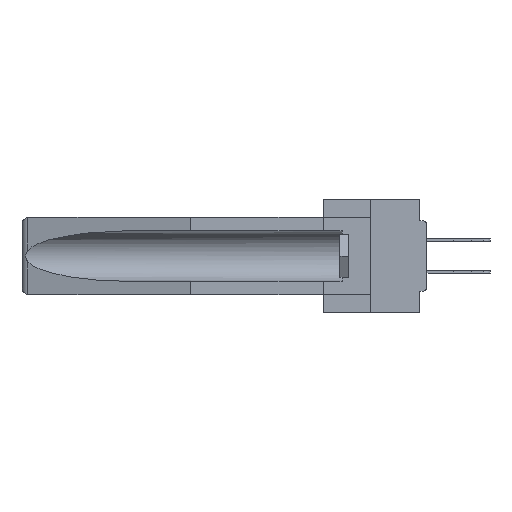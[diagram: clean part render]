
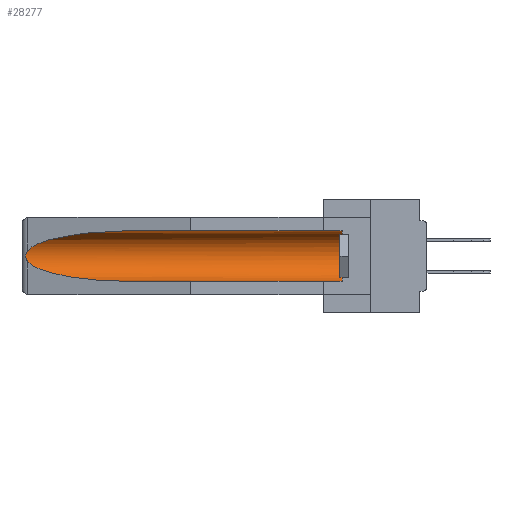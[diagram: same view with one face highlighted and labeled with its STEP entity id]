
A CAD part, left-side view. The second image highlights one B-rep face of the part: STEP entity #28277.
In plain terms, the highlighted cylindrical face has radius 2.857 mm (diameter 5.715 mm), a partial arc.
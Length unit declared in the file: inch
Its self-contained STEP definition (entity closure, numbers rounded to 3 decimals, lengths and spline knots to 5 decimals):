
#495 = ORIENTED_EDGE ( 'NONE', *, *, #36455, .T. ) ;
#780 = VERTEX_POINT ( 'NONE', #21716 ) ;
#1612 = CARTESIAN_POINT ( 'NONE',  ( 0.155, -0.30754, -0.1715 ) ) ;
#3388 = CARTESIAN_POINT ( 'NONE',  ( 0.26537, 1.52718, -0.14972 ) ) ;
#5120 = CARTESIAN_POINT ( 'NONE',  ( 0.155, 1.07973, -0.284 ) ) ;
#6222 = CYLINDRICAL_SURFACE ( 'NONE', #22054, 0.1125 ) ;
#7911 = CARTESIAN_POINT ( 'NONE',  ( 0.25451, 1.48313, -0.24835 ) ) ;
#8624 = CARTESIAN_POINT ( 'NONE',  ( 0.26654, 1.53092, -0.15636 ) ) ;
#9059 = CARTESIAN_POINT ( 'NONE',  ( 0.155, 1.07973, -0.284 ) ) ;
#9326 = VERTEX_POINT ( 'NONE', #36988 ) ;
#9457 = VERTEX_POINT ( 'NONE', #29042 ) ;
#10705 = EDGE_CURVE ( 'NONE', #15200, #37314, #19899, .T. ) ;
#11607 = VECTOR ( 'NONE', #16218, 39.37008 ) ;
#12542 = AXIS2_PLACEMENT_3D ( 'NONE', #43571, #39860, #30005 ) ;
#14572 = VECTOR ( 'NONE', #39892, 39.37008 ) ;
#15200 = VERTEX_POINT ( 'NONE', #37333 ) ;
#15576 = CARTESIAN_POINT ( 'NONE',  ( 0.2675, 1.53308, -0.16763 ) ) ;
#16218 = DIRECTION ( 'NONE',  ( 0., 1., 0. ) ) ;
#16695 = EDGE_CURVE ( 'NONE', #780, #9326, #34191, .T. ) ;
#19899 = B_SPLINE_CURVE_WITH_KNOTS ( 'NONE', 3,
 ( #35708, #32034, #8624, #36005, #15576, #36138, #23096, #43178, #22802, #39740 ),
 .UNSPECIFIED., .F., .F.,
 ( 4, 2, 2, 2, 4 ),
 ( 0., 0.00029, 0.00058, 0.00087, 0.00117 ),
 .UNSPECIFIED. ) ;
#20051 = CARTESIAN_POINT ( 'NONE',  ( 0.155, 1.07973, -0.059 ) ) ;
#21716 = CARTESIAN_POINT ( 'NONE',  ( 0.155, 0.126, -0.284 ) ) ;
#22054 = AXIS2_PLACEMENT_3D ( 'NONE', #1612, #22292, #28975 ) ;
#22292 = DIRECTION ( 'NONE',  ( 0., 1., 0. ) ) ;
#22752 = ORIENTED_EDGE ( 'NONE', *, *, #16695, .T. ) ;
#22802 = CARTESIAN_POINT ( 'NONE',  ( 0.26597, 1.5296, -0.19026 ) ) ;
#22813 = CARTESIAN_POINT ( 'NONE',  ( 0.21114, 1.30732, -0.284 ) ) ;
#23096 = CARTESIAN_POINT ( 'NONE',  ( 0.2673, 1.53269, -0.17917 ) ) ;
#24603 = VERTEX_POINT ( 'NONE', #5120 ) ;
#26087 = EDGE_CURVE ( 'NONE', #9457, #15200, #29199, .T. ) ;
#26638 = CARTESIAN_POINT ( 'NONE',  ( 0.155, -0.30754, -0.284 ) ) ;
#27066 = CARTESIAN_POINT ( 'NONE',  ( 0.21114, 1.30732, -0.059 ) ) ;
#28277 = ADVANCED_FACE ( 'NONE', ( #44075 ), #6222, .F. ) ;
#28849 = CARTESIAN_POINT ( 'NONE',  ( 0.26537, 1.52718, -0.19328 ) ) ;
#28975 = DIRECTION ( 'NONE',  ( 0., 0., 1. ) ) ;
#29028 = LINE ( 'NONE', #26638, #14572 ) ;
#29042 = CARTESIAN_POINT ( 'NONE',  ( 0.155, 1.07973, -0.059 ) ) ;
#29199 =( BOUNDED_CURVE ( )  B_SPLINE_CURVE ( 3, ( #20051, #27066, #37299, #3388 ),
 .UNSPECIFIED., .F., .F. ) 
 B_SPLINE_CURVE_WITH_KNOTS ( ( 4, 4 ),
 ( 4.71239, 6.08839 ),
 .UNSPECIFIED. ) 
 CURVE ( )  GEOMETRIC_REPRESENTATION_ITEM ( )  RATIONAL_B_SPLINE_CURVE ( ( 1., 0.848, 0.848, 1. ) ) 
 REPRESENTATION_ITEM ( '' )  );
#29481 = CARTESIAN_POINT ( 'NONE',  ( 0.26537, 1.52718, -0.19328 ) ) ;
#30005 = DIRECTION ( 'NONE',  ( 0., 0., 1. ) ) ;
#30096 = EDGE_CURVE ( 'NONE', #37314, #24603, #36533, .T. ) ;
#30276 = EDGE_CURVE ( 'NONE', #780, #24603, #29028, .T. ) ;
#30584 = EDGE_LOOP ( 'NONE', ( #32807, #31946, #38619, #37623, #22752, #495 ) ) ;
#31946 = ORIENTED_EDGE ( 'NONE', *, *, #10705, .T. ) ;
#32034 = CARTESIAN_POINT ( 'NONE',  ( 0.26597, 1.52961, -0.15275 ) ) ;
#32807 = ORIENTED_EDGE ( 'NONE', *, *, #26087, .T. ) ;
#33506 = CARTESIAN_POINT ( 'NONE',  ( 0.155, -0.30754, -0.059 ) ) ;
#34191 = CIRCLE ( 'NONE', #12542, 0.1125 ) ;
#35708 = CARTESIAN_POINT ( 'NONE',  ( 0.26537, 1.52718, -0.14972 ) ) ;
#36005 = CARTESIAN_POINT ( 'NONE',  ( 0.2673, 1.5327, -0.16383 ) ) ;
#36138 = CARTESIAN_POINT ( 'NONE',  ( 0.2675, 1.53308, -0.17534 ) ) ;
#36455 = EDGE_CURVE ( 'NONE', #9326, #9457, #37195, .T. ) ;
#36533 =( BOUNDED_CURVE ( )  B_SPLINE_CURVE ( 3, ( #29481, #7911, #22813, #9059 ),
 .UNSPECIFIED., .F., .F. ) 
 B_SPLINE_CURVE_WITH_KNOTS ( ( 4, 4 ),
 ( 0.1948, 1.5708 ),
 .UNSPECIFIED. ) 
 CURVE ( )  GEOMETRIC_REPRESENTATION_ITEM ( )  RATIONAL_B_SPLINE_CURVE ( ( 1., 0.848, 0.848, 1. ) ) 
 REPRESENTATION_ITEM ( '' )  );
#36988 = CARTESIAN_POINT ( 'NONE',  ( 0.155, 0.126, -0.059 ) ) ;
#37195 = LINE ( 'NONE', #33506, #11607 ) ;
#37299 = CARTESIAN_POINT ( 'NONE',  ( 0.25451, 1.48313, -0.09465 ) ) ;
#37314 = VERTEX_POINT ( 'NONE', #28849 ) ;
#37333 = CARTESIAN_POINT ( 'NONE',  ( 0.26537, 1.52718, -0.14972 ) ) ;
#37623 = ORIENTED_EDGE ( 'NONE', *, *, #30276, .F. ) ;
#38619 = ORIENTED_EDGE ( 'NONE', *, *, #30096, .T. ) ;
#39740 = CARTESIAN_POINT ( 'NONE',  ( 0.26537, 1.52718, -0.19328 ) ) ;
#39860 = DIRECTION ( 'NONE',  ( 0., -1., 0. ) ) ;
#39892 = DIRECTION ( 'NONE',  ( 0., 1., 0. ) ) ;
#43178 = CARTESIAN_POINT ( 'NONE',  ( 0.26655, 1.53094, -0.18657 ) ) ;
#43571 = CARTESIAN_POINT ( 'NONE',  ( 0.155, 0.126, -0.1715 ) ) ;
#44075 = FACE_OUTER_BOUND ( 'NONE', #30584, .T. ) ;
